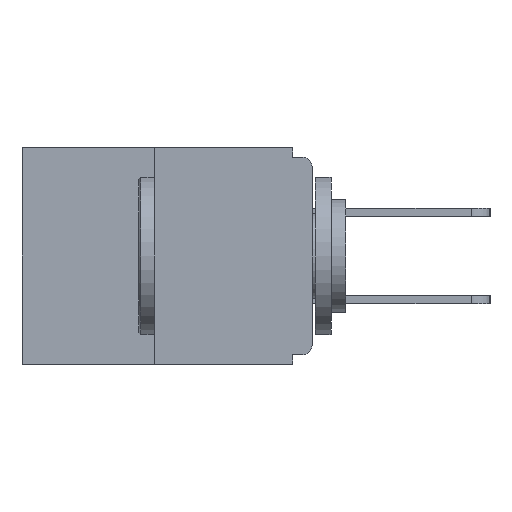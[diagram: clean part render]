
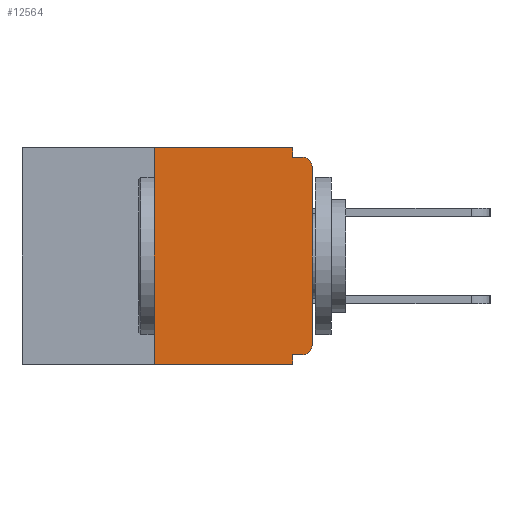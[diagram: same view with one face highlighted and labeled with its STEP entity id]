
A CAD part, left-side view. The second image highlights one B-rep face of the part: STEP entity #12564.
In plain terms, the highlighted planar face has unit normal (-1, 0, 0).
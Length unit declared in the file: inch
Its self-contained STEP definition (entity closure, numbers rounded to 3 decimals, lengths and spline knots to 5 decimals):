
#516 = LINE ( 'NONE', #13273, #16831 ) ;
#1258 = CARTESIAN_POINT ( 'NONE',  ( 0., 0.015, -0.03 ) ) ;
#1540 = VERTEX_POINT ( 'NONE', #10834 ) ;
#1806 = VERTEX_POINT ( 'NONE', #13110 ) ;
#1895 = LINE ( 'NONE', #7691, #16489 ) ;
#2012 = EDGE_CURVE ( 'NONE', #8280, #11695, #13349, .T. ) ;
#2047 = CIRCLE ( 'NONE', #12068, 0.015 ) ;
#2342 = LINE ( 'NONE', #14366, #14801 ) ;
#2818 = VERTEX_POINT ( 'NONE', #8381 ) ;
#2822 = EDGE_CURVE ( 'NONE', #1806, #6578, #13540, .T. ) ;
#3087 = CARTESIAN_POINT ( 'NONE',  ( 0., 0.46, -0.343 ) ) ;
#3506 = LINE ( 'NONE', #3087, #16820 ) ;
#3773 = EDGE_CURVE ( 'NONE', #11304, #15023, #8985, .T. ) ;
#5141 = ORIENTED_EDGE ( 'NONE', *, *, #8967, .T. ) ;
#5222 = VERTEX_POINT ( 'NONE', #9679 ) ;
#5269 = ORIENTED_EDGE ( 'NONE', *, *, #6144, .F. ) ;
#5969 = CARTESIAN_POINT ( 'NONE',  ( 0., 0.25, 0. ) ) ;
#6144 = EDGE_CURVE ( 'NONE', #11695, #1806, #516, .T. ) ;
#6487 = CARTESIAN_POINT ( 'NONE',  ( 0., 0., -0.015 ) ) ;
#6552 = ORIENTED_EDGE ( 'NONE', *, *, #14863, .F. ) ;
#6578 = VERTEX_POINT ( 'NONE', #7905 ) ;
#6640 = LINE ( 'NONE', #11899, #9844 ) ;
#6819 = DIRECTION ( 'NONE',  ( 0., 0., -1. ) ) ;
#6879 = DIRECTION ( 'NONE',  ( 1., 0., 0. ) ) ;
#6919 = ORIENTED_EDGE ( 'NONE', *, *, #10716, .T. ) ;
#7040 = ORIENTED_EDGE ( 'NONE', *, *, #2822, .F. ) ;
#7480 = EDGE_LOOP ( 'NONE', ( #5269, #7487, #12674, #11657, #6552, #12944, #5141, #6919, #8443, #7040 ) ) ;
#7487 = ORIENTED_EDGE ( 'NONE', *, *, #2012, .F. ) ;
#7565 = CARTESIAN_POINT ( 'NONE',  ( 0., 0.015, -0.328 ) ) ;
#7691 = CARTESIAN_POINT ( 'NONE',  ( 0., 0., 0. ) ) ;
#7884 = DIRECTION ( 'NONE',  ( 0., -1., 0. ) ) ;
#7905 = CARTESIAN_POINT ( 'NONE',  ( 0., 0.031, -0.015 ) ) ;
#7997 = DIRECTION ( 'NONE',  ( -1., 0., 0. ) ) ;
#8280 = VERTEX_POINT ( 'NONE', #16588 ) ;
#8320 = AXIS2_PLACEMENT_3D ( 'NONE', #14018, #16589, #9651 ) ;
#8381 = CARTESIAN_POINT ( 'NONE',  ( 0., 0., -0.03 ) ) ;
#8443 = ORIENTED_EDGE ( 'NONE', *, *, #17594, .F. ) ;
#8967 = EDGE_CURVE ( 'NONE', #15023, #2818, #1895, .T. ) ;
#8985 = CIRCLE ( 'NONE', #8320, 0.015 ) ;
#9651 = DIRECTION ( 'NONE',  ( 0., 0., -1. ) ) ;
#9679 = CARTESIAN_POINT ( 'NONE',  ( 0., 0.031, -0.328 ) ) ;
#9844 = VECTOR ( 'NONE', #13289, 39.37008 ) ;
#10162 = CARTESIAN_POINT ( 'NONE',  ( 0., 0.25, 0. ) ) ;
#10487 = DIRECTION ( 'NONE',  ( 0., -1., 0. ) ) ;
#10716 = EDGE_CURVE ( 'NONE', #2818, #12772, #2047, .T. ) ;
#10727 = VECTOR ( 'NONE', #7884, 39.37008 ) ;
#10734 = VECTOR ( 'NONE', #16694, 39.37008 ) ;
#10834 = CARTESIAN_POINT ( 'NONE',  ( 0., 0.031, -0.343 ) ) ;
#10850 = DIRECTION ( 'NONE',  ( 0., 0., -1. ) ) ;
#11183 = DIRECTION ( 'NONE',  ( 0., -1., 0. ) ) ;
#11227 = CARTESIAN_POINT ( 'NONE',  ( 0., 0.015, -0.015 ) ) ;
#11236 = DIRECTION ( 'NONE',  ( 0., 0., 1. ) ) ;
#11304 = VERTEX_POINT ( 'NONE', #7565 ) ;
#11657 = ORIENTED_EDGE ( 'NONE', *, *, #15092, .F. ) ;
#11695 = VERTEX_POINT ( 'NONE', #10162 ) ;
#11899 = CARTESIAN_POINT ( 'NONE',  ( 0., 0.031, -0.343 ) ) ;
#12068 = AXIS2_PLACEMENT_3D ( 'NONE', #1258, #7997, #10850 ) ;
#12098 = FACE_OUTER_BOUND ( 'NONE', #7480, .T. ) ;
#12266 = EDGE_CURVE ( 'NONE', #8280, #1540, #3506, .T. ) ;
#12564 = ADVANCED_FACE ( 'NONE', ( #12098 ), #15137, .F. ) ;
#12674 = ORIENTED_EDGE ( 'NONE', *, *, #12266, .T. ) ;
#12772 = VERTEX_POINT ( 'NONE', #11227 ) ;
#12944 = ORIENTED_EDGE ( 'NONE', *, *, #3773, .T. ) ;
#13110 = CARTESIAN_POINT ( 'NONE',  ( 0., 0.031, 0. ) ) ;
#13158 = CARTESIAN_POINT ( 'NONE',  ( 0., 0., -0.313 ) ) ;
#13273 = CARTESIAN_POINT ( 'NONE',  ( 0., 0.46, 0. ) ) ;
#13289 = DIRECTION ( 'NONE',  ( 0., 0., -1. ) ) ;
#13349 = LINE ( 'NONE', #5969, #14837 ) ;
#13540 = LINE ( 'NONE', #13938, #10734 ) ;
#13816 = LINE ( 'NONE', #6487, #10727 ) ;
#13938 = CARTESIAN_POINT ( 'NONE',  ( 0., 0.031, 0. ) ) ;
#14018 = CARTESIAN_POINT ( 'NONE',  ( 0., 0.015, -0.313 ) ) ;
#14366 = CARTESIAN_POINT ( 'NONE',  ( 0., 0., -0.328 ) ) ;
#14602 = AXIS2_PLACEMENT_3D ( 'NONE', #16207, #6879, #6819 ) ;
#14801 = VECTOR ( 'NONE', #17149, 39.37008 ) ;
#14837 = VECTOR ( 'NONE', #11236, 39.37008 ) ;
#14863 = EDGE_CURVE ( 'NONE', #11304, #5222, #2342, .T. ) ;
#15023 = VERTEX_POINT ( 'NONE', #13158 ) ;
#15092 = EDGE_CURVE ( 'NONE', #5222, #1540, #6640, .T. ) ;
#15137 = PLANE ( 'NONE',  #14602 ) ;
#16207 = CARTESIAN_POINT ( 'NONE',  ( 0., 0.46, 0. ) ) ;
#16489 = VECTOR ( 'NONE', #17128, 39.37008 ) ;
#16588 = CARTESIAN_POINT ( 'NONE',  ( 0., 0.25, -0.343 ) ) ;
#16589 = DIRECTION ( 'NONE',  ( -1., 0., 0. ) ) ;
#16694 = DIRECTION ( 'NONE',  ( 0., 0., -1. ) ) ;
#16820 = VECTOR ( 'NONE', #11183, 39.37008 ) ;
#16831 = VECTOR ( 'NONE', #10487, 39.37008 ) ;
#17128 = DIRECTION ( 'NONE',  ( 0., 0., 1. ) ) ;
#17149 = DIRECTION ( 'NONE',  ( 0., 1., 0. ) ) ;
#17594 = EDGE_CURVE ( 'NONE', #6578, #12772, #13816, .T. ) ;
